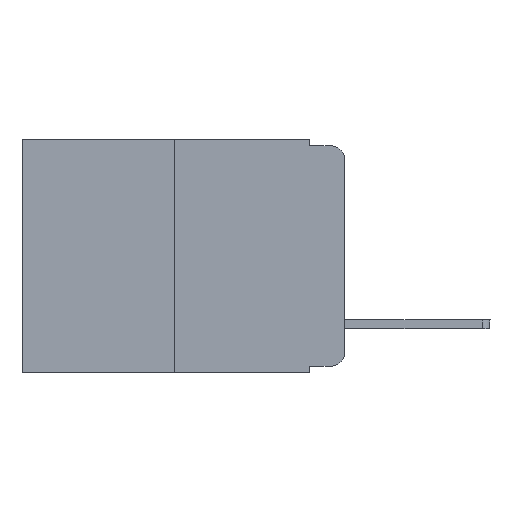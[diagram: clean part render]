
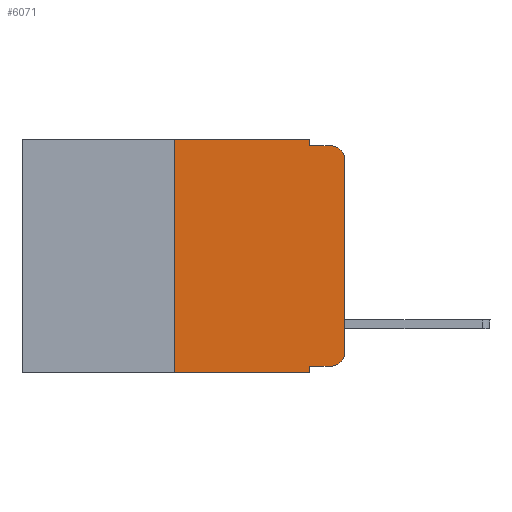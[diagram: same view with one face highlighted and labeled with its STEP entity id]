
A CAD part, left-side view. The second image highlights one B-rep face of the part: STEP entity #6071.
In plain terms, the highlighted planar face has unit normal (-1, 0, 0).
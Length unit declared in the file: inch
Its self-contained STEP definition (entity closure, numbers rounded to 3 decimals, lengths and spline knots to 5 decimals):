
#595 = VERTEX_POINT ( 'NONE', #21702 ) ;
#1028 = DIRECTION ( 'NONE',  ( -1., 0., 0. ) ) ;
#1180 = VECTOR ( 'NONE', #19068, 39.37008 ) ;
#1247 = VECTOR ( 'NONE', #3862, 39.37008 ) ;
#2021 = DIRECTION ( 'NONE',  ( 0., 0., -1. ) ) ;
#2159 = CARTESIAN_POINT ( 'NONE',  ( 0., 0.051, -0.01 ) ) ;
#2226 = VERTEX_POINT ( 'NONE', #15594 ) ;
#2557 = EDGE_CURVE ( 'NONE', #595, #8876, #5006, .T. ) ;
#2614 = EDGE_CURVE ( 'NONE', #8876, #9618, #16734, .T. ) ;
#2684 = ORIENTED_EDGE ( 'NONE', *, *, #14908, .T. ) ;
#3682 = CIRCLE ( 'NONE', #18443, 0.02 ) ;
#3708 = CARTESIAN_POINT ( 'NONE',  ( 0., 0.02, -0.03 ) ) ;
#3862 = DIRECTION ( 'NONE',  ( 0., 0., -1. ) ) ;
#4033 = CARTESIAN_POINT ( 'NONE',  ( 0., 0.051, -0.343 ) ) ;
#4456 = LINE ( 'NONE', #7901, #22931 ) ;
#4535 = EDGE_CURVE ( 'NONE', #21527, #10084, #20537, .T. ) ;
#4644 = CARTESIAN_POINT ( 'NONE',  ( 0., 0.02, -0.01 ) ) ;
#4662 = VECTOR ( 'NONE', #8643, 39.37008 ) ;
#5006 = LINE ( 'NONE', #19395, #14628 ) ;
#5055 = VERTEX_POINT ( 'NONE', #4644 ) ;
#5362 = AXIS2_PLACEMENT_3D ( 'NONE', #17406, #1028, #13457 ) ;
#5859 = PLANE ( 'NONE',  #11951 ) ;
#6071 = ADVANCED_FACE ( 'NONE', ( #23297 ), #5859, .F. ) ;
#6398 = CARTESIAN_POINT ( 'NONE',  ( 0., 0.25, 0. ) ) ;
#6785 = ORIENTED_EDGE ( 'NONE', *, *, #2614, .T. ) ;
#7749 = ORIENTED_EDGE ( 'NONE', *, *, #23093, .F. ) ;
#7901 = CARTESIAN_POINT ( 'NONE',  ( 0., 0., 0. ) ) ;
#8107 = CARTESIAN_POINT ( 'NONE',  ( 0., 0.473, 0. ) ) ;
#8643 = DIRECTION ( 'NONE',  ( 0., -1., 0. ) ) ;
#8812 = VECTOR ( 'NONE', #10984, 39.37008 ) ;
#8876 = VERTEX_POINT ( 'NONE', #14952 ) ;
#9267 = DIRECTION ( 'NONE',  ( 0., 0., -1. ) ) ;
#9558 = EDGE_CURVE ( 'NONE', #9618, #15550, #4456, .T. ) ;
#9618 = VERTEX_POINT ( 'NONE', #12510 ) ;
#10084 = VERTEX_POINT ( 'NONE', #4033 ) ;
#10118 = VERTEX_POINT ( 'NONE', #6398 ) ;
#10984 = DIRECTION ( 'NONE',  ( 0., 0., 1. ) ) ;
#11017 = LINE ( 'NONE', #25169, #1180 ) ;
#11652 = LINE ( 'NONE', #19712, #1247 ) ;
#11768 = DIRECTION ( 'NONE',  ( -1., 0., 0. ) ) ;
#11781 = VECTOR ( 'NONE', #22389, 39.37008 ) ;
#11951 = AXIS2_PLACEMENT_3D ( 'NONE', #8107, #22244, #2021 ) ;
#12046 = ORIENTED_EDGE ( 'NONE', *, *, #17531, .F. ) ;
#12510 = CARTESIAN_POINT ( 'NONE',  ( 0., 0., -0.313 ) ) ;
#13264 = CARTESIAN_POINT ( 'NONE',  ( 0., 0., -0.03 ) ) ;
#13292 = ORIENTED_EDGE ( 'NONE', *, *, #17291, .F. ) ;
#13457 = DIRECTION ( 'NONE',  ( 0., 0., -1. ) ) ;
#13819 = ORIENTED_EDGE ( 'NONE', *, *, #4535, .T. ) ;
#14323 = LINE ( 'NONE', #18665, #11781 ) ;
#14425 = LINE ( 'NONE', #2159, #22321 ) ;
#14565 = EDGE_LOOP ( 'NONE', ( #16521, #2684, #13292, #7749, #22814, #12046, #13819, #21226, #19012, #6785 ) ) ;
#14628 = VECTOR ( 'NONE', #21260, 39.37008 ) ;
#14908 = EDGE_CURVE ( 'NONE', #15550, #5055, #3682, .T. ) ;
#14952 = CARTESIAN_POINT ( 'NONE',  ( 0., 0.02, -0.333 ) ) ;
#15550 = VERTEX_POINT ( 'NONE', #13264 ) ;
#15594 = CARTESIAN_POINT ( 'NONE',  ( 0., 0.051, 0. ) ) ;
#15612 = CARTESIAN_POINT ( 'NONE',  ( 0., 0.051, -0.01 ) ) ;
#15645 = EDGE_CURVE ( 'NONE', #595, #10084, #11017, .T. ) ;
#15949 = DIRECTION ( 'NONE',  ( 0., 0., 1. ) ) ;
#16521 = ORIENTED_EDGE ( 'NONE', *, *, #9558, .T. ) ;
#16734 = CIRCLE ( 'NONE', #5362, 0.02 ) ;
#17291 = EDGE_CURVE ( 'NONE', #19901, #5055, #14425, .T. ) ;
#17406 = CARTESIAN_POINT ( 'NONE',  ( 0., 0.02, -0.313 ) ) ;
#17531 = EDGE_CURVE ( 'NONE', #21527, #10118, #19038, .T. ) ;
#18443 = AXIS2_PLACEMENT_3D ( 'NONE', #3708, #11768, #9267 ) ;
#18665 = CARTESIAN_POINT ( 'NONE',  ( 0., 0.473, 0. ) ) ;
#19012 = ORIENTED_EDGE ( 'NONE', *, *, #2557, .T. ) ;
#19038 = LINE ( 'NONE', #21030, #8812 ) ;
#19068 = DIRECTION ( 'NONE',  ( 0., 0., -1. ) ) ;
#19395 = CARTESIAN_POINT ( 'NONE',  ( 0., 0.051, -0.333 ) ) ;
#19712 = CARTESIAN_POINT ( 'NONE',  ( 0., 0.051, 0. ) ) ;
#19901 = VERTEX_POINT ( 'NONE', #15612 ) ;
#20537 = LINE ( 'NONE', #20921, #4662 ) ;
#20921 = CARTESIAN_POINT ( 'NONE',  ( 0., 0.473, -0.343 ) ) ;
#21030 = CARTESIAN_POINT ( 'NONE',  ( 0., 0.25, 0. ) ) ;
#21226 = ORIENTED_EDGE ( 'NONE', *, *, #15645, .F. ) ;
#21260 = DIRECTION ( 'NONE',  ( 0., -1., 0. ) ) ;
#21527 = VERTEX_POINT ( 'NONE', #25415 ) ;
#21702 = CARTESIAN_POINT ( 'NONE',  ( 0., 0.051, -0.333 ) ) ;
#22244 = DIRECTION ( 'NONE',  ( 1., 0., 0. ) ) ;
#22321 = VECTOR ( 'NONE', #24232, 39.37008 ) ;
#22389 = DIRECTION ( 'NONE',  ( 0., -1., 0. ) ) ;
#22750 = EDGE_CURVE ( 'NONE', #10118, #2226, #14323, .T. ) ;
#22814 = ORIENTED_EDGE ( 'NONE', *, *, #22750, .F. ) ;
#22931 = VECTOR ( 'NONE', #15949, 39.37008 ) ;
#23093 = EDGE_CURVE ( 'NONE', #2226, #19901, #11652, .T. ) ;
#23297 = FACE_OUTER_BOUND ( 'NONE', #14565, .T. ) ;
#24232 = DIRECTION ( 'NONE',  ( 0., -1., 0. ) ) ;
#25169 = CARTESIAN_POINT ( 'NONE',  ( 0., 0.051, 0. ) ) ;
#25415 = CARTESIAN_POINT ( 'NONE',  ( 0., 0.25, -0.343 ) ) ;
